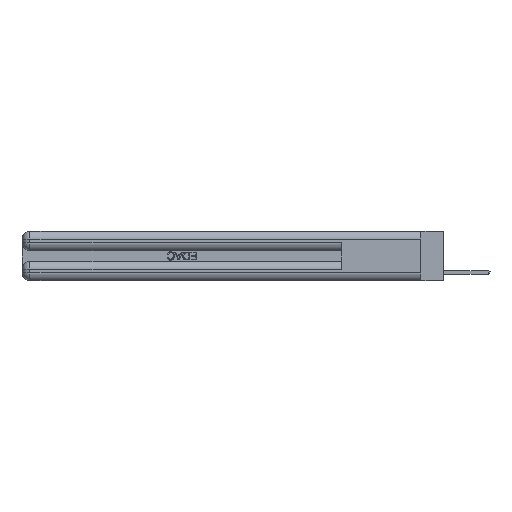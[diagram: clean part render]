
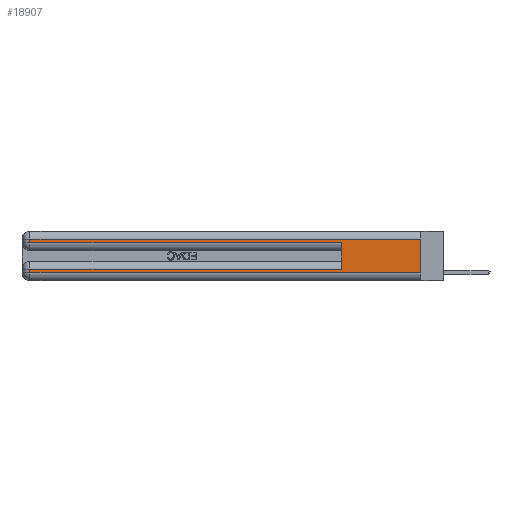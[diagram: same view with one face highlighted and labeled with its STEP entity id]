
A CAD part, left-side view. The second image highlights one B-rep face of the part: STEP entity #18907.
In plain terms, the highlighted planar face has unit normal (-1, 0, 0).
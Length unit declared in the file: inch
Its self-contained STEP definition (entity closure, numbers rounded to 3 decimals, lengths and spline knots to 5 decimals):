
#588 = ORIENTED_EDGE ( 'NONE', *, *, #13534, .T. ) ;
#973 = VERTEX_POINT ( 'NONE', #21548 ) ;
#1151 = LINE ( 'NONE', #4495, #18743 ) ;
#1437 = VECTOR ( 'NONE', #3375, 39.37008 ) ;
#1516 = CARTESIAN_POINT ( 'NONE',  ( 0., 0., 0.31 ) ) ;
#2019 = VERTEX_POINT ( 'NONE', #2634 ) ;
#2074 = CARTESIAN_POINT ( 'NONE',  ( 0., 2.94, 0.06 ) ) ;
#2634 = CARTESIAN_POINT ( 'NONE',  ( 0., 2.94, 0.31 ) ) ;
#2747 = EDGE_CURVE ( 'NONE', #14891, #21738, #4901, .T. ) ;
#3375 = DIRECTION ( 'NONE',  ( 0., 0., -1. ) ) ;
#3550 = PLANE ( 'NONE',  #22258 ) ;
#4495 = CARTESIAN_POINT ( 'NONE',  ( 0., 0., 0.37 ) ) ;
#4577 = CARTESIAN_POINT ( 'NONE',  ( 0., 0., 0.285 ) ) ;
#4901 = LINE ( 'NONE', #23831, #18876 ) ;
#5450 = CARTESIAN_POINT ( 'NONE',  ( 0., 0.6, 0.285 ) ) ;
#5492 = DIRECTION ( 'NONE',  ( 0., 0., -1. ) ) ;
#5551 = EDGE_CURVE ( 'NONE', #19383, #12706, #11401, .T. ) ;
#5670 = CARTESIAN_POINT ( 'NONE',  ( 0., 0., 0.37 ) ) ;
#6744 = ORIENTED_EDGE ( 'NONE', *, *, #21126, .F. ) ;
#7557 = ORIENTED_EDGE ( 'NONE', *, *, #15222, .T. ) ;
#7590 = EDGE_LOOP ( 'NONE', ( #9353, #14921, #7557, #19622, #6744, #10175, #588, #14899 ) ) ;
#7883 = EDGE_CURVE ( 'NONE', #21499, #24789, #9639, .T. ) ;
#9353 = ORIENTED_EDGE ( 'NONE', *, *, #11250, .F. ) ;
#9639 = LINE ( 'NONE', #22093, #14636 ) ;
#9737 = VECTOR ( 'NONE', #26041, 39.37008 ) ;
#10109 = VECTOR ( 'NONE', #22327, 39.37008 ) ;
#10175 = ORIENTED_EDGE ( 'NONE', *, *, #7883, .T. ) ;
#10974 = DIRECTION ( 'NONE',  ( 0., -1., 0. ) ) ;
#11071 = LINE ( 'NONE', #12005, #1437 ) ;
#11218 = CARTESIAN_POINT ( 'NONE',  ( 0., 2.94, 0.285 ) ) ;
#11250 = EDGE_CURVE ( 'NONE', #973, #21738, #1151, .T. ) ;
#11401 = LINE ( 'NONE', #4577, #24744 ) ;
#11462 = LINE ( 'NONE', #20084, #10109 ) ;
#12005 = CARTESIAN_POINT ( 'NONE',  ( 0., 2.94, 0.37 ) ) ;
#12706 = VERTEX_POINT ( 'NONE', #5450 ) ;
#13534 = EDGE_CURVE ( 'NONE', #24789, #14891, #11462, .T. ) ;
#14215 = DIRECTION ( 'NONE',  ( 1., 0., 0. ) ) ;
#14636 = VECTOR ( 'NONE', #15478, 39.37008 ) ;
#14891 = VERTEX_POINT ( 'NONE', #2074 ) ;
#14899 = ORIENTED_EDGE ( 'NONE', *, *, #2747, .T. ) ;
#14921 = ORIENTED_EDGE ( 'NONE', *, *, #15317, .T. ) ;
#15206 = CARTESIAN_POINT ( 'NONE',  ( 0., 0.6, 0.145 ) ) ;
#15222 = EDGE_CURVE ( 'NONE', #2019, #19383, #11071, .T. ) ;
#15317 = EDGE_CURVE ( 'NONE', #973, #2019, #16728, .T. ) ;
#15478 = DIRECTION ( 'NONE',  ( 0., 1., 0. ) ) ;
#15922 = DIRECTION ( 'NONE',  ( 0., 0., -1. ) ) ;
#16371 = DIRECTION ( 'NONE',  ( 0., 1., 0. ) ) ;
#16497 = FACE_OUTER_BOUND ( 'NONE', #7590, .T. ) ;
#16728 = LINE ( 'NONE', #1516, #23721 ) ;
#16882 = CARTESIAN_POINT ( 'NONE',  ( 0., 0.6, 0.085 ) ) ;
#17706 = LINE ( 'NONE', #15206, #9737 ) ;
#18743 = VECTOR ( 'NONE', #15922, 39.37008 ) ;
#18876 = VECTOR ( 'NONE', #20457, 39.37008 ) ;
#18907 = ADVANCED_FACE ( 'NONE', ( #16497 ), #3550, .F. ) ;
#19383 = VERTEX_POINT ( 'NONE', #11218 ) ;
#19622 = ORIENTED_EDGE ( 'NONE', *, *, #5551, .T. ) ;
#19914 = CARTESIAN_POINT ( 'NONE',  ( 0., 2.94, 0.085 ) ) ;
#20084 = CARTESIAN_POINT ( 'NONE',  ( 0., 2.94, 0.37 ) ) ;
#20457 = DIRECTION ( 'NONE',  ( 0., -1., 0. ) ) ;
#21126 = EDGE_CURVE ( 'NONE', #21499, #12706, #17706, .T. ) ;
#21499 = VERTEX_POINT ( 'NONE', #16882 ) ;
#21548 = CARTESIAN_POINT ( 'NONE',  ( 0., 0., 0.31 ) ) ;
#21738 = VERTEX_POINT ( 'NONE', #24386 ) ;
#22093 = CARTESIAN_POINT ( 'NONE',  ( 0., 0., 0.085 ) ) ;
#22258 = AXIS2_PLACEMENT_3D ( 'NONE', #5670, #14215, #5492 ) ;
#22327 = DIRECTION ( 'NONE',  ( 0., 0., -1. ) ) ;
#23721 = VECTOR ( 'NONE', #16371, 39.37008 ) ;
#23831 = CARTESIAN_POINT ( 'NONE',  ( 0., 0., 0.06 ) ) ;
#24386 = CARTESIAN_POINT ( 'NONE',  ( 0., 0., 0.06 ) ) ;
#24744 = VECTOR ( 'NONE', #10974, 39.37008 ) ;
#24789 = VERTEX_POINT ( 'NONE', #19914 ) ;
#26041 = DIRECTION ( 'NONE',  ( 0., 0., 1. ) ) ;
